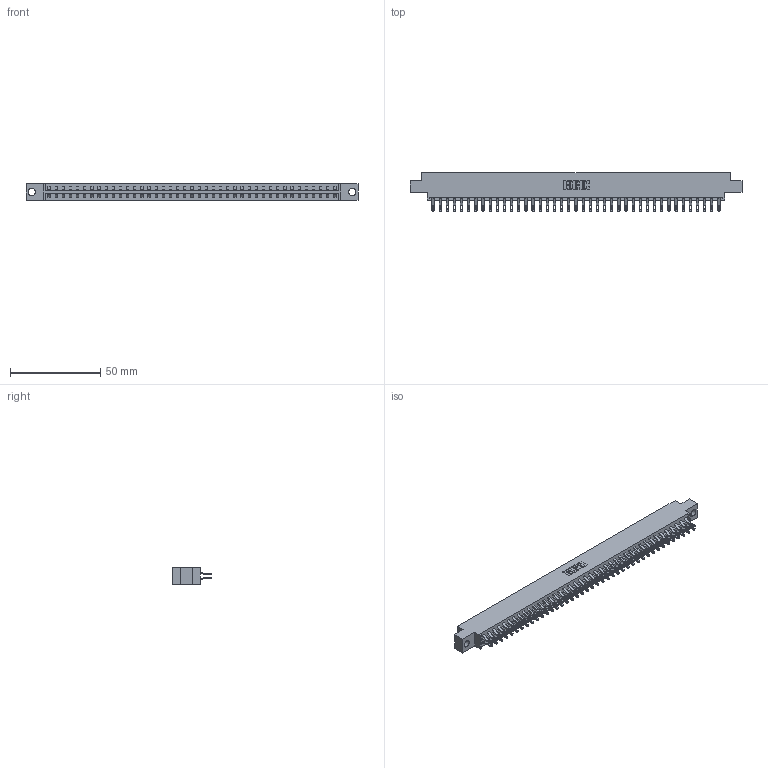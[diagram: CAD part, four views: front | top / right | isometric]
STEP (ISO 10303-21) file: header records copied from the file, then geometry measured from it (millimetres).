
FILE_DESCRIPTION (( 'STEP AP203' ), '1' );
FILE_NAME ('333-082-555-804.STEP', '2018-08-05T03:27:09', ( '' ), ( '' ), 'SwSTEP 2.0', 'SolidWorks 2016', '' );
FILE_SCHEMA (( 'CONFIG_CONTROL_DESIGN' ));
Length unit declared in the file: inch
Products named in the file (3): 333 Part_Offset - .156 Dia - TH; 345-292-001_555 Tail; 333-082-555-804
Assembly tree (83 placements, depth 2):
  333-082-555-804
    333 Part_Offset - .156 Dia - TH
    345-292-001_555 Tail  x82
Bounding box: 184 x 21.47 x 9.4 mm (x, y, z)
Volume: 18697.9 mm3; surface area: 23004.6 mm2
Topology: 83 solids, 83 shells, 4874 faces, 15329 edges, 10218 vertices
Faces by surface type: plane 2862, cylinder 2012
Entity records: 26967 total; most frequent: CARTESIAN_POINT 4508, ORIENTED_EDGE 4414, DIRECTION 3823, EDGE_CURVE 2207, LINE 2059, VECTOR 2059, VERTEX_POINT 1470, AXIS2_PLACEMENT_3D 882
